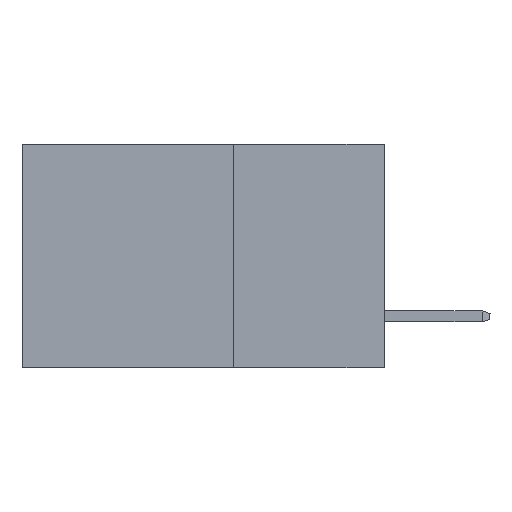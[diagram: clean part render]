
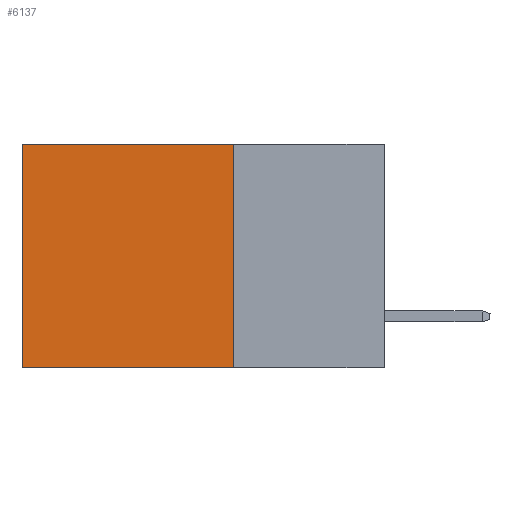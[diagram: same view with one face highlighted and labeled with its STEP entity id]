
A CAD part, left-side view. The second image highlights one B-rep face of the part: STEP entity #6137.
In plain terms, the highlighted planar face has unit normal (-1, 0, 0).
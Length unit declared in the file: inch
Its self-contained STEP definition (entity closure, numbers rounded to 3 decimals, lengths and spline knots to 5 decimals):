
#1203 = VECTOR ( 'NONE', #12349, 39.37008 ) ;
#1998 = CARTESIAN_POINT ( 'NONE',  ( 0.2615, 0.25, -0.37 ) ) ;
#2874 = FACE_OUTER_BOUND ( 'NONE', #5203, .T. ) ;
#3082 = EDGE_CURVE ( 'NONE', #9322, #11883, #3226, .T. ) ;
#3158 = DIRECTION ( 'NONE',  ( 0., 1., 0. ) ) ;
#3190 = EDGE_CURVE ( 'NONE', #12097, #6221, #7444, .T. ) ;
#3226 = LINE ( 'NONE', #10202, #4796 ) ;
#3354 = ORIENTED_EDGE ( 'NONE', *, *, #10557, .F. ) ;
#3408 = DIRECTION ( 'NONE',  ( 1., 0., 0. ) ) ;
#4159 = LINE ( 'NONE', #9311, #1203 ) ;
#4796 = VECTOR ( 'NONE', #3158, 39.37008 ) ;
#4869 = EDGE_CURVE ( 'NONE', #6221, #11883, #4159, .T. ) ;
#5086 = DIRECTION ( 'NONE',  ( 0., 0., -1. ) ) ;
#5203 = EDGE_LOOP ( 'NONE', ( #12173, #12258, #3354, #10162 ) ) ;
#6137 = ADVANCED_FACE ( 'NONE', ( #2874 ), #6977, .F. ) ;
#6221 = VERTEX_POINT ( 'NONE', #6431 ) ;
#6360 = CARTESIAN_POINT ( 'NONE',  ( 0.2615, 0.25, 0. ) ) ;
#6373 = CARTESIAN_POINT ( 'NONE',  ( 0.2615, 0.25, -0.37 ) ) ;
#6431 = CARTESIAN_POINT ( 'NONE',  ( 0.2615, 0.6, 0. ) ) ;
#6505 = DIRECTION ( 'NONE',  ( 0., 0., -1. ) ) ;
#6977 = PLANE ( 'NONE',  #8510 ) ;
#7444 = LINE ( 'NONE', #10464, #12554 ) ;
#8510 = AXIS2_PLACEMENT_3D ( 'NONE', #1998, #3408, #6505 ) ;
#8886 = CARTESIAN_POINT ( 'NONE',  ( 0.2615, 0.25, -0.37 ) ) ;
#9311 = CARTESIAN_POINT ( 'NONE',  ( 0.2615, 0.6, -0.37 ) ) ;
#9322 = VERTEX_POINT ( 'NONE', #8886 ) ;
#9692 = VECTOR ( 'NONE', #5086, 39.37008 ) ;
#9974 = CARTESIAN_POINT ( 'NONE',  ( 0.2615, 0.6, -0.37 ) ) ;
#10162 = ORIENTED_EDGE ( 'NONE', *, *, #3190, .T. ) ;
#10202 = CARTESIAN_POINT ( 'NONE',  ( 0.2615, 0.25, -0.37 ) ) ;
#10464 = CARTESIAN_POINT ( 'NONE',  ( 0.2615, 0.25, 0. ) ) ;
#10557 = EDGE_CURVE ( 'NONE', #12097, #9322, #11480, .T. ) ;
#11480 = LINE ( 'NONE', #6373, #9692 ) ;
#11499 = DIRECTION ( 'NONE',  ( 0., 1., 0. ) ) ;
#11883 = VERTEX_POINT ( 'NONE', #9974 ) ;
#12097 = VERTEX_POINT ( 'NONE', #6360 ) ;
#12173 = ORIENTED_EDGE ( 'NONE', *, *, #4869, .T. ) ;
#12258 = ORIENTED_EDGE ( 'NONE', *, *, #3082, .F. ) ;
#12349 = DIRECTION ( 'NONE',  ( 0., 0., -1. ) ) ;
#12554 = VECTOR ( 'NONE', #11499, 39.37008 ) ;
